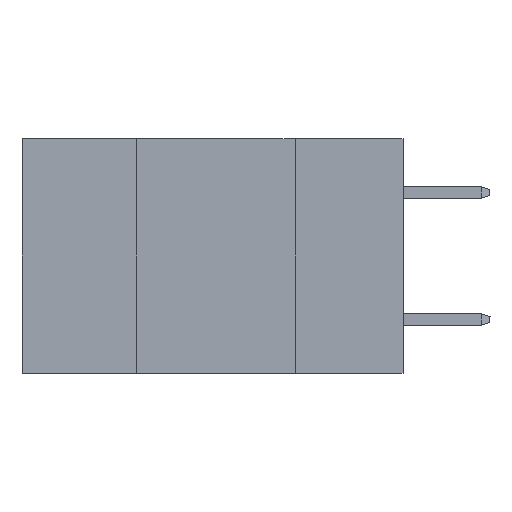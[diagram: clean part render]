
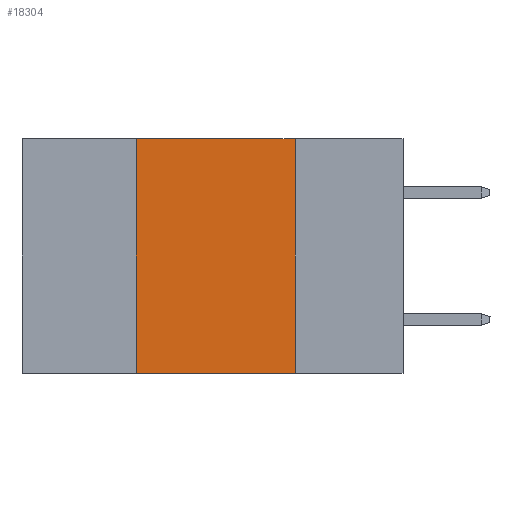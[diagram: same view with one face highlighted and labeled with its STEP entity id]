
A CAD part, left-side view. The second image highlights one B-rep face of the part: STEP entity #18304.
In plain terms, the highlighted planar face has unit normal (-1, 0, 0).
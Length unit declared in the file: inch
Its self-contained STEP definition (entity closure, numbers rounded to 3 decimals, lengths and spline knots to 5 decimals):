
#351 = VECTOR ( 'NONE', #8415, 39.37008 ) ;
#676 = DIRECTION ( 'NONE',  ( 0., 0., -1. ) ) ;
#1588 = VECTOR ( 'NONE', #21662, 39.37008 ) ;
#1629 = CARTESIAN_POINT ( 'NONE',  ( 0., 0.42, 0. ) ) ;
#1794 = DIRECTION ( 'NONE',  ( 0., 0., -1. ) ) ;
#1985 = CARTESIAN_POINT ( 'NONE',  ( 0., 0.17, 0. ) ) ;
#1987 = ORIENTED_EDGE ( 'NONE', *, *, #9593, .F. ) ;
#3581 = LINE ( 'NONE', #18062, #7677 ) ;
#4331 = PLANE ( 'NONE',  #15110 ) ;
#4346 = EDGE_CURVE ( 'NONE', #6978, #14667, #15663, .T. ) ;
#4362 = CARTESIAN_POINT ( 'NONE',  ( 0., 0.6, -0.37 ) ) ;
#4473 = DIRECTION ( 'NONE',  ( 0., -1., 0. ) ) ;
#6978 = VERTEX_POINT ( 'NONE', #11982 ) ;
#7677 = VECTOR ( 'NONE', #1794, 39.37008 ) ;
#8415 = DIRECTION ( 'NONE',  ( 0., 0., 1. ) ) ;
#8647 = VERTEX_POINT ( 'NONE', #11531 ) ;
#9593 = EDGE_CURVE ( 'NONE', #14667, #12750, #17893, .T. ) ;
#10071 = EDGE_CURVE ( 'NONE', #12750, #8647, #3581, .T. ) ;
#10559 = ORIENTED_EDGE ( 'NONE', *, *, #4346, .F. ) ;
#10850 = ORIENTED_EDGE ( 'NONE', *, *, #10071, .F. ) ;
#10926 = CARTESIAN_POINT ( 'NONE',  ( 0., 0.42, 0. ) ) ;
#11531 = CARTESIAN_POINT ( 'NONE',  ( 0., 0.17, -0.37 ) ) ;
#11982 = CARTESIAN_POINT ( 'NONE',  ( 0., 0.42, -0.37 ) ) ;
#12700 = EDGE_LOOP ( 'NONE', ( #10850, #1987, #10559, #17974 ) ) ;
#12750 = VERTEX_POINT ( 'NONE', #1985 ) ;
#12963 = VECTOR ( 'NONE', #4473, 39.37008 ) ;
#14667 = VERTEX_POINT ( 'NONE', #10926 ) ;
#15110 = AXIS2_PLACEMENT_3D ( 'NONE', #16958, #19069, #676 ) ;
#15173 = FACE_OUTER_BOUND ( 'NONE', #12700, .T. ) ;
#15663 = LINE ( 'NONE', #1629, #351 ) ;
#16958 = CARTESIAN_POINT ( 'NONE',  ( 0., 0.6, 0. ) ) ;
#17893 = LINE ( 'NONE', #18341, #1588 ) ;
#17974 = ORIENTED_EDGE ( 'NONE', *, *, #23014, .T. ) ;
#18062 = CARTESIAN_POINT ( 'NONE',  ( 0., 0.17, 0. ) ) ;
#18304 = ADVANCED_FACE ( 'NONE', ( #15173 ), #4331, .F. ) ;
#18341 = CARTESIAN_POINT ( 'NONE',  ( 0., 0.6, 0. ) ) ;
#19069 = DIRECTION ( 'NONE',  ( 1., 0., 0. ) ) ;
#21662 = DIRECTION ( 'NONE',  ( 0., -1., 0. ) ) ;
#22159 = LINE ( 'NONE', #4362, #12963 ) ;
#23014 = EDGE_CURVE ( 'NONE', #6978, #8647, #22159, .T. ) ;
